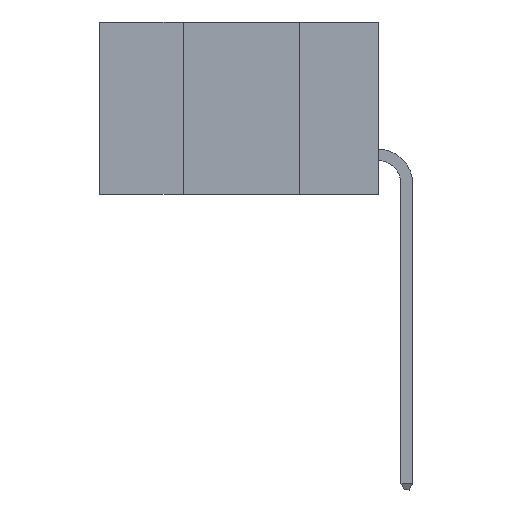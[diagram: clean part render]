
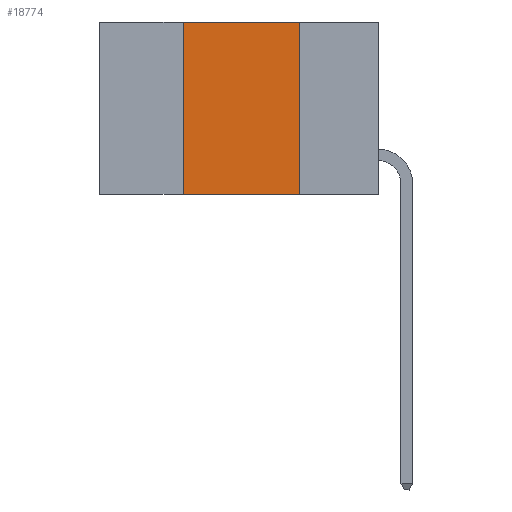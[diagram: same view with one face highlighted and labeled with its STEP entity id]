
A CAD part, left-side view. The second image highlights one B-rep face of the part: STEP entity #18774.
In plain terms, the highlighted planar face has unit normal (-1, 0, 0).
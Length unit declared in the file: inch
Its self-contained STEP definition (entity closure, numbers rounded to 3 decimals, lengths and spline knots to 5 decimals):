
#89 = VECTOR ( 'NONE', #5676, 39.37008 ) ;
#103 = CARTESIAN_POINT ( 'NONE',  ( 0., 0.42, 0. ) ) ;
#318 = ORIENTED_EDGE ( 'NONE', *, *, #571, .F. ) ;
#571 = EDGE_CURVE ( 'NONE', #1934, #9348, #14001, .T. ) ;
#1641 = DIRECTION ( 'NONE',  ( 1., 0., 0. ) ) ;
#1934 = VERTEX_POINT ( 'NONE', #19252 ) ;
#3716 = VECTOR ( 'NONE', #14357, 39.37008 ) ;
#3762 = EDGE_CURVE ( 'NONE', #9062, #1934, #8362, .T. ) ;
#5273 = CARTESIAN_POINT ( 'NONE',  ( 0., 0.17, 0. ) ) ;
#5339 = AXIS2_PLACEMENT_3D ( 'NONE', #12078, #1641, #13843 ) ;
#5676 = DIRECTION ( 'NONE',  ( 0., 0., -1. ) ) ;
#5952 = LINE ( 'NONE', #103, #14015 ) ;
#6871 = PLANE ( 'NONE',  #5339 ) ;
#8362 = LINE ( 'NONE', #14132, #3716 ) ;
#8942 = DIRECTION ( 'NONE',  ( 0., 0., 1. ) ) ;
#9062 = VERTEX_POINT ( 'NONE', #16819 ) ;
#9113 = ORIENTED_EDGE ( 'NONE', *, *, #21664, .F. ) ;
#9348 = VERTEX_POINT ( 'NONE', #17525 ) ;
#9438 = LINE ( 'NONE', #16482, #17988 ) ;
#9631 = DIRECTION ( 'NONE',  ( 0., -1., 0. ) ) ;
#10938 = CARTESIAN_POINT ( 'NONE',  ( 0., 0.42, -0.37 ) ) ;
#12078 = CARTESIAN_POINT ( 'NONE',  ( 0., 0.6, 0. ) ) ;
#12622 = ORIENTED_EDGE ( 'NONE', *, *, #16155, .T. ) ;
#12895 = ORIENTED_EDGE ( 'NONE', *, *, #3762, .F. ) ;
#12991 = EDGE_LOOP ( 'NONE', ( #318, #12895, #9113, #12622 ) ) ;
#13843 = DIRECTION ( 'NONE',  ( 0., 0., -1. ) ) ;
#14001 = LINE ( 'NONE', #5273, #89 ) ;
#14015 = VECTOR ( 'NONE', #8942, 39.37008 ) ;
#14132 = CARTESIAN_POINT ( 'NONE',  ( 0., 0.6, 0. ) ) ;
#14357 = DIRECTION ( 'NONE',  ( 0., -1., 0. ) ) ;
#15008 = FACE_OUTER_BOUND ( 'NONE', #12991, .T. ) ;
#15303 = VERTEX_POINT ( 'NONE', #10938 ) ;
#16155 = EDGE_CURVE ( 'NONE', #15303, #9348, #9438, .T. ) ;
#16482 = CARTESIAN_POINT ( 'NONE',  ( 0., 0.6, -0.37 ) ) ;
#16819 = CARTESIAN_POINT ( 'NONE',  ( 0., 0.42, 0. ) ) ;
#17525 = CARTESIAN_POINT ( 'NONE',  ( 0., 0.17, -0.37 ) ) ;
#17988 = VECTOR ( 'NONE', #9631, 39.37008 ) ;
#18774 = ADVANCED_FACE ( 'NONE', ( #15008 ), #6871, .F. ) ;
#19252 = CARTESIAN_POINT ( 'NONE',  ( 0., 0.17, 0. ) ) ;
#21664 = EDGE_CURVE ( 'NONE', #15303, #9062, #5952, .T. ) ;
